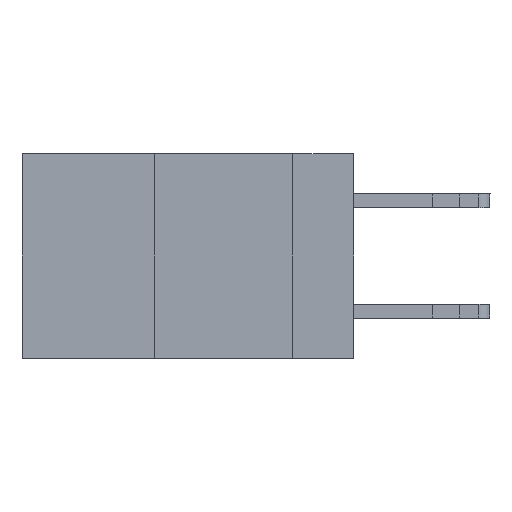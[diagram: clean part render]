
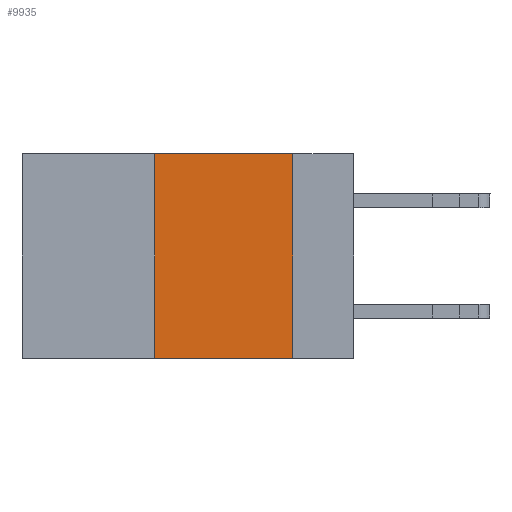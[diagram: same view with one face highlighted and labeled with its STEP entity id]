
A CAD part, left-side view. The second image highlights one B-rep face of the part: STEP entity #9935.
In plain terms, the highlighted planar face has unit normal (-1, 0, 0).
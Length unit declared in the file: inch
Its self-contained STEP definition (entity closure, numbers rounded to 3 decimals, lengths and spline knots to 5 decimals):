
#942 = ORIENTED_EDGE ( 'NONE', *, *, #18229, .F. ) ;
#958 = LINE ( 'NONE', #26618, #7886 ) ;
#1224 = DIRECTION ( 'NONE',  ( 1., 0., 0. ) ) ;
#1793 = CARTESIAN_POINT ( 'NONE',  ( 0., 0.36, -0.37 ) ) ;
#3423 = CARTESIAN_POINT ( 'NONE',  ( 0., 0.36, 0. ) ) ;
#4570 = CARTESIAN_POINT ( 'NONE',  ( 0., 0.11, -0.37 ) ) ;
#4581 = VECTOR ( 'NONE', #18697, 39.37008 ) ;
#5062 = DIRECTION ( 'NONE',  ( 0., 0., 1. ) ) ;
#5477 = CARTESIAN_POINT ( 'NONE',  ( 0., 0.6, -0.37 ) ) ;
#5989 = EDGE_CURVE ( 'NONE', #14324, #16803, #27163, .T. ) ;
#6892 = LINE ( 'NONE', #22022, #20975 ) ;
#7886 = VECTOR ( 'NONE', #14348, 39.37008 ) ;
#8236 = VERTEX_POINT ( 'NONE', #3423 ) ;
#8873 = LINE ( 'NONE', #14676, #4581 ) ;
#9935 = ADVANCED_FACE ( 'NONE', ( #24798 ), #11793, .F. ) ;
#11793 = PLANE ( 'NONE',  #20617 ) ;
#13266 = ORIENTED_EDGE ( 'NONE', *, *, #23211, .F. ) ;
#14324 = VERTEX_POINT ( 'NONE', #1793 ) ;
#14348 = DIRECTION ( 'NONE',  ( 0., -1., 0. ) ) ;
#14419 = ORIENTED_EDGE ( 'NONE', *, *, #23959, .F. ) ;
#14676 = CARTESIAN_POINT ( 'NONE',  ( 0., 0.11, 0. ) ) ;
#16228 = ORIENTED_EDGE ( 'NONE', *, *, #5989, .T. ) ;
#16803 = VERTEX_POINT ( 'NONE', #4570 ) ;
#17309 = VECTOR ( 'NONE', #24164, 39.37008 ) ;
#17957 = CARTESIAN_POINT ( 'NONE',  ( 0., 0.6, 0. ) ) ;
#18229 = EDGE_CURVE ( 'NONE', #14324, #8236, #6892, .T. ) ;
#18697 = DIRECTION ( 'NONE',  ( 0., 0., -1. ) ) ;
#20617 = AXIS2_PLACEMENT_3D ( 'NONE', #17957, #1224, #22326 ) ;
#20975 = VECTOR ( 'NONE', #5062, 39.37008 ) ;
#21210 = CARTESIAN_POINT ( 'NONE',  ( 0., 0.11, 0. ) ) ;
#21911 = EDGE_LOOP ( 'NONE', ( #14419, #13266, #942, #16228 ) ) ;
#22022 = CARTESIAN_POINT ( 'NONE',  ( 0., 0.36, 0. ) ) ;
#22326 = DIRECTION ( 'NONE',  ( 0., 0., -1. ) ) ;
#23211 = EDGE_CURVE ( 'NONE', #8236, #25388, #958, .T. ) ;
#23959 = EDGE_CURVE ( 'NONE', #25388, #16803, #8873, .T. ) ;
#24164 = DIRECTION ( 'NONE',  ( 0., -1., 0. ) ) ;
#24798 = FACE_OUTER_BOUND ( 'NONE', #21911, .T. ) ;
#25388 = VERTEX_POINT ( 'NONE', #21210 ) ;
#26618 = CARTESIAN_POINT ( 'NONE',  ( 0., 0.6, 0. ) ) ;
#27163 = LINE ( 'NONE', #5477, #17309 ) ;
